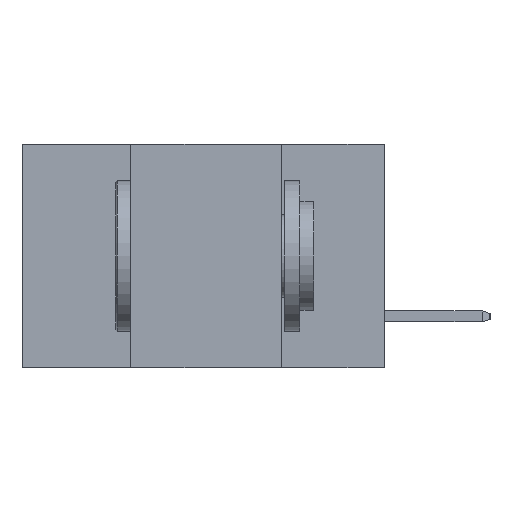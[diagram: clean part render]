
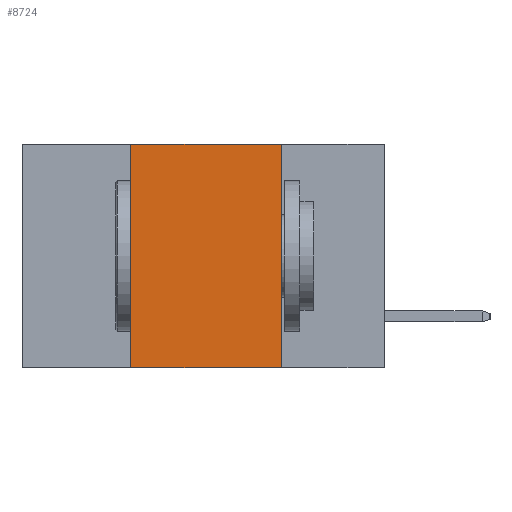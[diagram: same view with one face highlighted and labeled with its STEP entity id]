
A CAD part, left-side view. The second image highlights one B-rep face of the part: STEP entity #8724.
In plain terms, the highlighted planar face has unit normal (-1, 0, 0).
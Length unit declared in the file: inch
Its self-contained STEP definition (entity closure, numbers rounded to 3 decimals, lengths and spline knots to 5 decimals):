
#33 = AXIS2_PLACEMENT_3D ( 'NONE', #7266, #3682, #12076 ) ;
#68 = LINE ( 'NONE', #7695, #6210 ) ;
#415 = VERTEX_POINT ( 'NONE', #3258 ) ;
#1042 = EDGE_CURVE ( 'NONE', #10056, #415, #3926, .T. ) ;
#1218 = PLANE ( 'NONE',  #33 ) ;
#1751 = ORIENTED_EDGE ( 'NONE', *, *, #1042, .T. ) ;
#1841 = EDGE_CURVE ( 'NONE', #10056, #8984, #68, .T. ) ;
#1902 = ORIENTED_EDGE ( 'NONE', *, *, #1841, .F. ) ;
#2658 = EDGE_CURVE ( 'NONE', #8984, #8754, #10103, .T. ) ;
#2956 = CARTESIAN_POINT ( 'NONE',  ( 0., 0.17, -0.37 ) ) ;
#3119 = DIRECTION ( 'NONE',  ( 0., -1., 0. ) ) ;
#3258 = CARTESIAN_POINT ( 'NONE',  ( 0., 0.17, -0.37 ) ) ;
#3327 = ORIENTED_EDGE ( 'NONE', *, *, #5129, .F. ) ;
#3368 = CARTESIAN_POINT ( 'NONE',  ( 0., 0.6, 0. ) ) ;
#3682 = DIRECTION ( 'NONE',  ( 1., 0., 0. ) ) ;
#3697 = DIRECTION ( 'NONE',  ( 0., -1., 0. ) ) ;
#3713 = VECTOR ( 'NONE', #3119, 39.37008 ) ;
#3728 = ORIENTED_EDGE ( 'NONE', *, *, #2658, .F. ) ;
#3894 = EDGE_LOOP ( 'NONE', ( #3327, #3728, #1902, #1751 ) ) ;
#3926 = LINE ( 'NONE', #10468, #9577 ) ;
#4176 = DIRECTION ( 'NONE',  ( 0., 0., 1. ) ) ;
#4319 = CARTESIAN_POINT ( 'NONE',  ( 0., 0.17, 0. ) ) ;
#4651 = FACE_OUTER_BOUND ( 'NONE', #3894, .T. ) ;
#5129 = EDGE_CURVE ( 'NONE', #8754, #415, #9079, .T. ) ;
#6210 = VECTOR ( 'NONE', #4176, 39.37008 ) ;
#7266 = CARTESIAN_POINT ( 'NONE',  ( 0., 0.6, 0. ) ) ;
#7661 = CARTESIAN_POINT ( 'NONE',  ( 0., 0.42, 0. ) ) ;
#7695 = CARTESIAN_POINT ( 'NONE',  ( 0., 0.42, -0.37 ) ) ;
#8702 = VECTOR ( 'NONE', #9403, 39.37008 ) ;
#8724 = ADVANCED_FACE ( 'NONE', ( #4651 ), #1218, .F. ) ;
#8754 = VERTEX_POINT ( 'NONE', #4319 ) ;
#8984 = VERTEX_POINT ( 'NONE', #7661 ) ;
#9079 = LINE ( 'NONE', #2956, #8702 ) ;
#9403 = DIRECTION ( 'NONE',  ( 0., 0., -1. ) ) ;
#9577 = VECTOR ( 'NONE', #3697, 39.37008 ) ;
#9882 = CARTESIAN_POINT ( 'NONE',  ( 0., 0.42, -0.37 ) ) ;
#10056 = VERTEX_POINT ( 'NONE', #9882 ) ;
#10103 = LINE ( 'NONE', #3368, #3713 ) ;
#10468 = CARTESIAN_POINT ( 'NONE',  ( 0., 0.6, -0.37 ) ) ;
#12076 = DIRECTION ( 'NONE',  ( 0., 0., -1. ) ) ;
